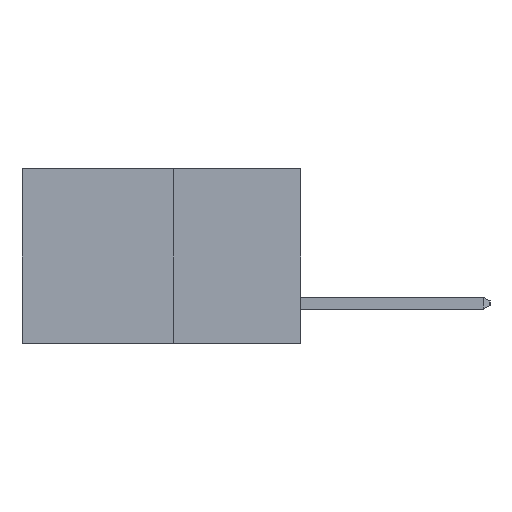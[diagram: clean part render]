
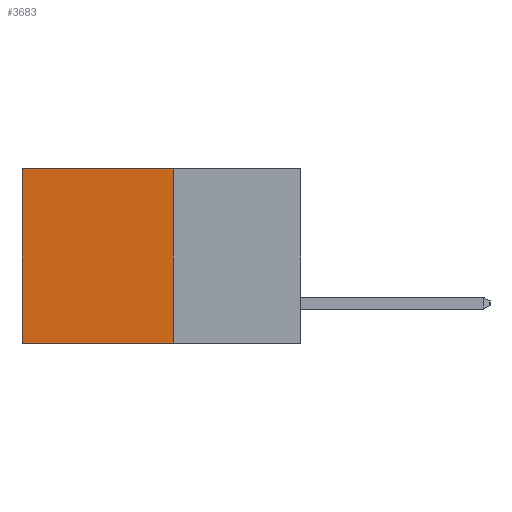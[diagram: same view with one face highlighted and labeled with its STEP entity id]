
A CAD part, left-side view. The second image highlights one B-rep face of the part: STEP entity #3683.
In plain terms, the highlighted planar face has unit normal (-1, 0, 0).
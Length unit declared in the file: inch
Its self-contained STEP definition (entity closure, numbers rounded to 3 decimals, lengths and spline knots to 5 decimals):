
#267 = LINE ( 'NONE', #16762, #17488 ) ;
#916 = DIRECTION ( 'NONE',  ( 0., 0., -1. ) ) ;
#1503 = VERTEX_POINT ( 'NONE', #16663 ) ;
#2460 = EDGE_CURVE ( 'NONE', #10155, #1503, #3352, .T. ) ;
#2780 = CARTESIAN_POINT ( 'NONE',  ( 0.277, 0.27, -0.37 ) ) ;
#3352 = LINE ( 'NONE', #2780, #16498 ) ;
#3683 = ADVANCED_FACE ( 'NONE', ( #8917 ), #7110, .F. ) ;
#3700 = EDGE_CURVE ( 'NONE', #1503, #4142, #267, .T. ) ;
#4142 = VERTEX_POINT ( 'NONE', #12117 ) ;
#6105 = EDGE_LOOP ( 'NONE', ( #15576, #16503, #10683, #21566 ) ) ;
#6294 = EDGE_CURVE ( 'NONE', #11869, #4142, #21632, .T. ) ;
#7110 = PLANE ( 'NONE',  #20728 ) ;
#8095 = LINE ( 'NONE', #17318, #21498 ) ;
#8917 = FACE_OUTER_BOUND ( 'NONE', #6105, .T. ) ;
#10155 = VERTEX_POINT ( 'NONE', #18010 ) ;
#10683 = ORIENTED_EDGE ( 'NONE', *, *, #2460, .F. ) ;
#11006 = CARTESIAN_POINT ( 'NONE',  ( 0.277, 0.27, -0.37 ) ) ;
#11869 = VERTEX_POINT ( 'NONE', #16643 ) ;
#12117 = CARTESIAN_POINT ( 'NONE',  ( 0.277, 0.59, -0.37 ) ) ;
#12311 = DIRECTION ( 'NONE',  ( 0., 1., 0. ) ) ;
#12671 = VECTOR ( 'NONE', #15839, 39.37008 ) ;
#15357 = CARTESIAN_POINT ( 'NONE',  ( 0.277, 0.59, -0.37 ) ) ;
#15576 = ORIENTED_EDGE ( 'NONE', *, *, #6294, .T. ) ;
#15839 = DIRECTION ( 'NONE',  ( 0., 0., -1. ) ) ;
#16498 = VECTOR ( 'NONE', #916, 39.37008 ) ;
#16503 = ORIENTED_EDGE ( 'NONE', *, *, #3700, .F. ) ;
#16643 = CARTESIAN_POINT ( 'NONE',  ( 0.277, 0.59, 0. ) ) ;
#16663 = CARTESIAN_POINT ( 'NONE',  ( 0.277, 0.27, -0.37 ) ) ;
#16762 = CARTESIAN_POINT ( 'NONE',  ( 0.277, 0.27, -0.37 ) ) ;
#17318 = CARTESIAN_POINT ( 'NONE',  ( 0.277, 0.27, 0. ) ) ;
#17407 = DIRECTION ( 'NONE',  ( 0., 0., -1. ) ) ;
#17488 = VECTOR ( 'NONE', #21688, 39.37008 ) ;
#18010 = CARTESIAN_POINT ( 'NONE',  ( 0.277, 0.27, 0. ) ) ;
#19588 = DIRECTION ( 'NONE',  ( 1., 0., 0. ) ) ;
#20728 = AXIS2_PLACEMENT_3D ( 'NONE', #11006, #19588, #17407 ) ;
#21498 = VECTOR ( 'NONE', #12311, 39.37008 ) ;
#21566 = ORIENTED_EDGE ( 'NONE', *, *, #21617, .T. ) ;
#21617 = EDGE_CURVE ( 'NONE', #10155, #11869, #8095, .T. ) ;
#21632 = LINE ( 'NONE', #15357, #12671 ) ;
#21688 = DIRECTION ( 'NONE',  ( 0., 1., 0. ) ) ;
